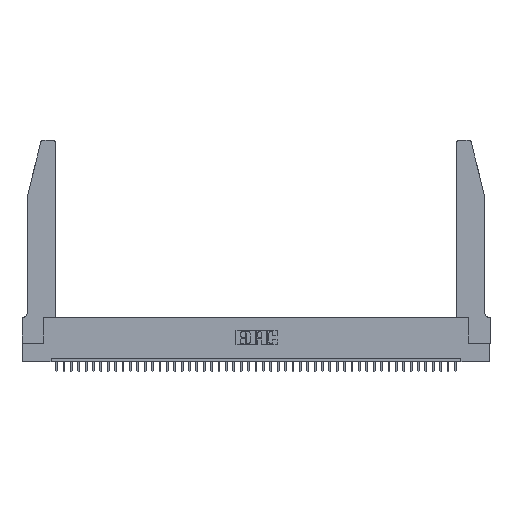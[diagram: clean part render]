
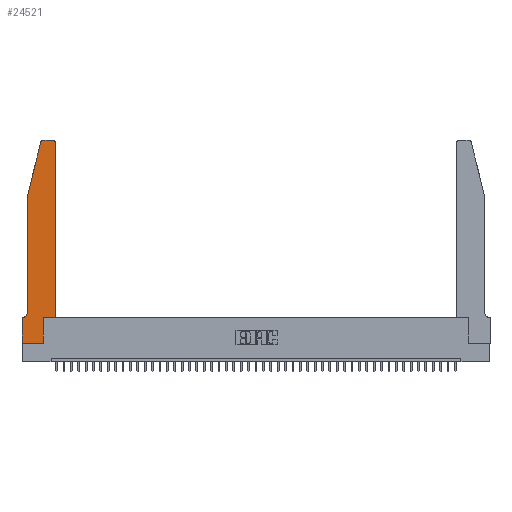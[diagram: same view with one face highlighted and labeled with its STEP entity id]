
A CAD part, top view. The second image highlights one B-rep face of the part: STEP entity #24521.
In plain terms, the highlighted planar face has unit normal (0, 0, 1).
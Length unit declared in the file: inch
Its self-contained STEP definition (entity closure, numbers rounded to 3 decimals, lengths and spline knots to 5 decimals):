
#68 = EDGE_CURVE ( 'NONE', #24213, #6436, #29162, .T. ) ;
#245 = VECTOR ( 'NONE', #15509, 39.37008 ) ;
#1388 = EDGE_CURVE ( 'NONE', #40564, #27496, #14466, .T. ) ;
#1977 = CARTESIAN_POINT ( 'NONE',  ( 0.0755, 2., 0.37 ) ) ;
#2566 = VERTEX_POINT ( 'NONE', #13025 ) ;
#2627 = CARTESIAN_POINT ( 'NONE',  ( 0.4505, 0.35, 0.37 ) ) ;
#2633 = AXIS2_PLACEMENT_3D ( 'NONE', #37789, #24320, #27811 ) ;
#3404 = LINE ( 'NONE', #9407, #35009 ) ;
#4436 = ORIENTED_EDGE ( 'NONE', *, *, #26799, .T. ) ;
#4543 = ORIENTED_EDGE ( 'NONE', *, *, #15037, .T. ) ;
#5174 = DIRECTION ( 'NONE',  ( 0., 1., 0. ) ) ;
#5785 = DIRECTION ( 'NONE',  ( -1., 0., 0. ) ) ;
#5829 = CARTESIAN_POINT ( 'NONE',  ( 0., 0.35, 0.37 ) ) ;
#5956 = VECTOR ( 'NONE', #7736, 39.37008 ) ;
#6436 = VERTEX_POINT ( 'NONE', #17743 ) ;
#6820 = ORIENTED_EDGE ( 'NONE', *, *, #31258, .T. ) ;
#7128 = ORIENTED_EDGE ( 'NONE', *, *, #19936, .T. ) ;
#7662 = FACE_OUTER_BOUND ( 'NONE', #31230, .T. ) ;
#7736 = DIRECTION ( 'NONE',  ( -1., 0., 0. ) ) ;
#7834 = DIRECTION ( 'NONE',  ( 1., 0., 0. ) ) ;
#9068 = EDGE_CURVE ( 'NONE', #10510, #42560, #34756, .T. ) ;
#9109 = CARTESIAN_POINT ( 'NONE',  ( 0.4205, 2.72, 0.37 ) ) ;
#9243 = DIRECTION ( 'NONE',  ( 1., 0., 0. ) ) ;
#9407 = CARTESIAN_POINT ( 'NONE',  ( 0.2865, 0.35, 0.37 ) ) ;
#9888 = CARTESIAN_POINT ( 'NONE',  ( 0.0755, 2., 0.37 ) ) ;
#9926 = AXIS2_PLACEMENT_3D ( 'NONE', #9109, #15992, #12576 ) ;
#9978 = LINE ( 'NONE', #25729, #245 ) ;
#10331 = VERTEX_POINT ( 'NONE', #19656 ) ;
#10367 = VERTEX_POINT ( 'NONE', #21560 ) ;
#10510 = VERTEX_POINT ( 'NONE', #2627 ) ;
#10559 = DIRECTION ( 'NONE',  ( 1., 0., 0. ) ) ;
#11486 = CARTESIAN_POINT ( 'NONE',  ( 0.4505, 0.35, 0.37 ) ) ;
#11696 = VECTOR ( 'NONE', #9243, 39.37008 ) ;
#12576 = DIRECTION ( 'NONE',  ( 1., 0., 0. ) ) ;
#13025 = CARTESIAN_POINT ( 'NONE',  ( 0.0055, 0.35, 0.37 ) ) ;
#13512 = ORIENTED_EDGE ( 'NONE', *, *, #26848, .T. ) ;
#13692 = EDGE_CURVE ( 'NONE', #2566, #24213, #20429, .T. ) ;
#13829 = CARTESIAN_POINT ( 'NONE',  ( 0., 0.35, 0.37 ) ) ;
#14097 = VECTOR ( 'NONE', #20891, 39.37008 ) ;
#14099 = VECTOR ( 'NONE', #24399, 39.37008 ) ;
#14466 = LINE ( 'NONE', #34738, #5956 ) ;
#14779 = ORIENTED_EDGE ( 'NONE', *, *, #39115, .T. ) ;
#15037 = EDGE_CURVE ( 'NONE', #27496, #36683, #30469, .T. ) ;
#15509 = DIRECTION ( 'NONE',  ( 1., 0., 0. ) ) ;
#15688 = DIRECTION ( 'NONE',  ( 0., 1., 0. ) ) ;
#15866 = EDGE_CURVE ( 'NONE', #42560, #40564, #30373, .T. ) ;
#15992 = DIRECTION ( 'NONE',  ( 0., 0., 1. ) ) ;
#17743 = CARTESIAN_POINT ( 'NONE',  ( 0., 0., 0.37 ) ) ;
#18151 = VECTOR ( 'NONE', #24306, 39.37008 ) ;
#18607 = CARTESIAN_POINT ( 'NONE',  ( 0.2865, 0.35, 0.37 ) ) ;
#19231 = LINE ( 'NONE', #1977, #18151 ) ;
#19306 = VECTOR ( 'NONE', #5785, 39.37008 ) ;
#19414 = CARTESIAN_POINT ( 'NONE',  ( 0., 0., 0.37 ) ) ;
#19656 = CARTESIAN_POINT ( 'NONE',  ( 0.0755, 0.42, 0.37 ) ) ;
#19936 = EDGE_CURVE ( 'NONE', #36683, #34760, #33442, .T. ) ;
#20429 = LINE ( 'NONE', #29356, #19306 ) ;
#20569 = CARTESIAN_POINT ( 'NONE',  ( 0.4205, 2.75, 0.37 ) ) ;
#20874 = CARTESIAN_POINT ( 'NONE',  ( 0.0755, 2., 0.37 ) ) ;
#20891 = DIRECTION ( 'NONE',  ( 0., -1., 0. ) ) ;
#21560 = CARTESIAN_POINT ( 'NONE',  ( 0.2865, 0., 0.37 ) ) ;
#22359 = VECTOR ( 'NONE', #5174, 39.37008 ) ;
#24213 = VERTEX_POINT ( 'NONE', #13829 ) ;
#24306 = DIRECTION ( 'NONE',  ( 0., -1., 0. ) ) ;
#24320 = DIRECTION ( 'NONE',  ( 0., 0., -1. ) ) ;
#24399 = DIRECTION ( 'NONE',  ( -0.239, -0.971, 0. ) ) ;
#24521 = ADVANCED_FACE ( 'NONE', ( #7662 ), #43574, .T. ) ;
#25729 = CARTESIAN_POINT ( 'NONE',  ( 0.4505, 0.35, 0.37 ) ) ;
#26799 = EDGE_CURVE ( 'NONE', #6436, #10367, #29956, .T. ) ;
#26848 = EDGE_CURVE ( 'NONE', #34760, #10331, #19231, .T. ) ;
#27188 = AXIS2_PLACEMENT_3D ( 'NONE', #5829, #29838, #10559 ) ;
#27496 = VERTEX_POINT ( 'NONE', #33067 ) ;
#27596 = ORIENTED_EDGE ( 'NONE', *, *, #68, .T. ) ;
#27811 = DIRECTION ( 'NONE',  ( -1., 0., 0. ) ) ;
#29162 = LINE ( 'NONE', #19414, #14097 ) ;
#29356 = CARTESIAN_POINT ( 'NONE',  ( 0.0755, 0.35, 0.37 ) ) ;
#29838 = DIRECTION ( 'NONE',  ( 0., 0., 1. ) ) ;
#29956 = LINE ( 'NONE', #43097, #11696 ) ;
#30373 = CIRCLE ( 'NONE', #9926, 0.03 ) ;
#30443 = CARTESIAN_POINT ( 'NONE',  ( 0.4505, 2.72, 0.37 ) ) ;
#30469 = CIRCLE ( 'NONE', #34020, 0.03 ) ;
#30913 = ORIENTED_EDGE ( 'NONE', *, *, #1388, .T. ) ;
#31230 = EDGE_LOOP ( 'NONE', ( #30913, #4543, #7128, #13512, #41966, #41673, #27596, #4436, #14779, #6820, #38802, #36078 ) ) ;
#31258 = EDGE_CURVE ( 'NONE', #34862, #10510, #9978, .T. ) ;
#33067 = CARTESIAN_POINT ( 'NONE',  ( 0.284, 2.75, 0.37 ) ) ;
#33442 = LINE ( 'NONE', #9888, #14099 ) ;
#34020 = AXIS2_PLACEMENT_3D ( 'NONE', #38852, #35270, #7834 ) ;
#34738 = CARTESIAN_POINT ( 'NONE',  ( 0.2605, 2.75, 0.37 ) ) ;
#34756 = LINE ( 'NONE', #11486, #22359 ) ;
#34760 = VERTEX_POINT ( 'NONE', #20874 ) ;
#34862 = VERTEX_POINT ( 'NONE', #18607 ) ;
#35009 = VECTOR ( 'NONE', #15688, 39.37008 ) ;
#35270 = DIRECTION ( 'NONE',  ( 0., 0., 1. ) ) ;
#36078 = ORIENTED_EDGE ( 'NONE', *, *, #15866, .T. ) ;
#36683 = VERTEX_POINT ( 'NONE', #43767 ) ;
#37789 = CARTESIAN_POINT ( 'NONE',  ( 0.0055, 0.42, 0.37 ) ) ;
#38802 = ORIENTED_EDGE ( 'NONE', *, *, #9068, .T. ) ;
#38852 = CARTESIAN_POINT ( 'NONE',  ( 0.284, 2.72, 0.37 ) ) ;
#39115 = EDGE_CURVE ( 'NONE', #10367, #34862, #3404, .T. ) ;
#40564 = VERTEX_POINT ( 'NONE', #20569 ) ;
#41673 = ORIENTED_EDGE ( 'NONE', *, *, #13692, .T. ) ;
#41726 = EDGE_CURVE ( 'NONE', #10331, #2566, #42285, .T. ) ;
#41966 = ORIENTED_EDGE ( 'NONE', *, *, #41726, .T. ) ;
#42285 = CIRCLE ( 'NONE', #2633, 0.07 ) ;
#42560 = VERTEX_POINT ( 'NONE', #30443 ) ;
#43097 = CARTESIAN_POINT ( 'NONE',  ( 0., 0., 0.37 ) ) ;
#43574 = PLANE ( 'NONE',  #27188 ) ;
#43767 = CARTESIAN_POINT ( 'NONE',  ( 0.25487, 2.72718, 0.37 ) ) ;
